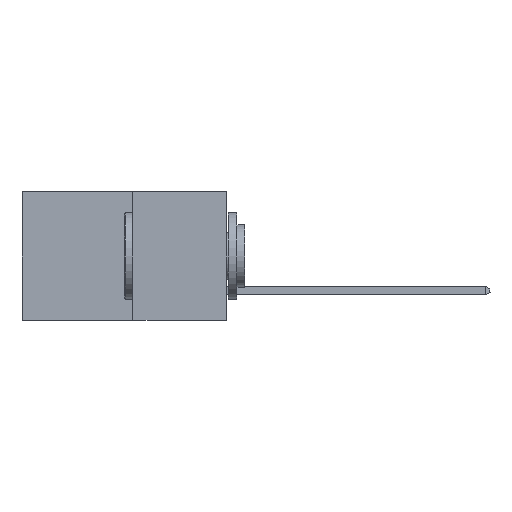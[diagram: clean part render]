
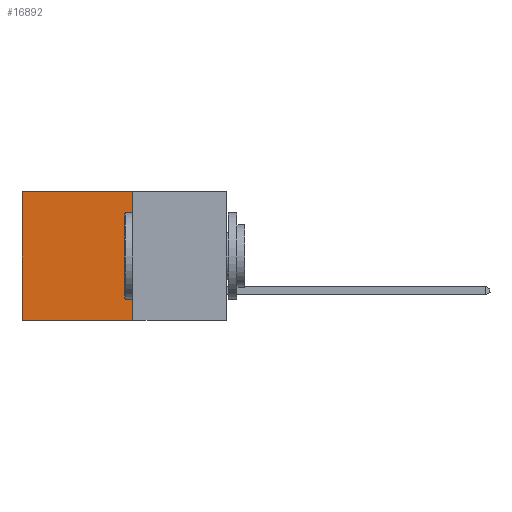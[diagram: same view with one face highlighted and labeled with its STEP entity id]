
A CAD part, left-side view. The second image highlights one B-rep face of the part: STEP entity #16892.
In plain terms, the highlighted planar face has unit normal (-1, 0, 0).
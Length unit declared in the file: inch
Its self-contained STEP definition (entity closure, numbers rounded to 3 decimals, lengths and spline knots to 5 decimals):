
#365 = VECTOR ( 'NONE', #19151, 39.37008 ) ;
#368 = CARTESIAN_POINT ( 'NONE',  ( 0.277, 0.59, 0. ) ) ;
#751 = FACE_OUTER_BOUND ( 'NONE', #15248, .T. ) ;
#902 = LINE ( 'NONE', #19407, #365 ) ;
#994 = CARTESIAN_POINT ( 'NONE',  ( 0.277, 0.27, -0.37 ) ) ;
#2076 = ORIENTED_EDGE ( 'NONE', *, *, #5922, .T. ) ;
#2740 = VECTOR ( 'NONE', #10110, 39.37008 ) ;
#2936 = CARTESIAN_POINT ( 'NONE',  ( 0.277, 0.59, -0.37 ) ) ;
#3285 = LINE ( 'NONE', #11860, #2740 ) ;
#3890 = LINE ( 'NONE', #19130, #8025 ) ;
#3902 = VERTEX_POINT ( 'NONE', #368 ) ;
#4713 = DIRECTION ( 'NONE',  ( 0., 0., -1. ) ) ;
#5631 = PLANE ( 'NONE',  #19453 ) ;
#5729 = VECTOR ( 'NONE', #4713, 39.37008 ) ;
#5922 = EDGE_CURVE ( 'NONE', #9801, #3902, #902, .T. ) ;
#7409 = DIRECTION ( 'NONE',  ( 1., 0., 0. ) ) ;
#7413 = VERTEX_POINT ( 'NONE', #19163 ) ;
#8025 = VECTOR ( 'NONE', #12296, 39.37008 ) ;
#8832 = VERTEX_POINT ( 'NONE', #994 ) ;
#9571 = EDGE_CURVE ( 'NONE', #3902, #7413, #10359, .T. ) ;
#9782 = ORIENTED_EDGE ( 'NONE', *, *, #15269, .F. ) ;
#9801 = VERTEX_POINT ( 'NONE', #20812 ) ;
#10110 = DIRECTION ( 'NONE',  ( 0., 1., 0. ) ) ;
#10359 = LINE ( 'NONE', #2936, #5729 ) ;
#10508 = ORIENTED_EDGE ( 'NONE', *, *, #9571, .T. ) ;
#11860 = CARTESIAN_POINT ( 'NONE',  ( 0.277, 0.27, -0.37 ) ) ;
#12296 = DIRECTION ( 'NONE',  ( 0., 0., -1. ) ) ;
#14237 = EDGE_CURVE ( 'NONE', #9801, #8832, #3890, .T. ) ;
#15248 = EDGE_LOOP ( 'NONE', ( #10508, #9782, #19873, #2076 ) ) ;
#15269 = EDGE_CURVE ( 'NONE', #8832, #7413, #3285, .T. ) ;
#16892 = ADVANCED_FACE ( 'NONE', ( #751 ), #5631, .F. ) ;
#17751 = CARTESIAN_POINT ( 'NONE',  ( 0.277, 0.27, -0.37 ) ) ;
#19130 = CARTESIAN_POINT ( 'NONE',  ( 0.277, 0.27, -0.37 ) ) ;
#19151 = DIRECTION ( 'NONE',  ( 0., 1., 0. ) ) ;
#19163 = CARTESIAN_POINT ( 'NONE',  ( 0.277, 0.59, -0.37 ) ) ;
#19407 = CARTESIAN_POINT ( 'NONE',  ( 0.277, 0.27, 0. ) ) ;
#19445 = DIRECTION ( 'NONE',  ( 0., 0., -1. ) ) ;
#19453 = AXIS2_PLACEMENT_3D ( 'NONE', #17751, #7409, #19445 ) ;
#19873 = ORIENTED_EDGE ( 'NONE', *, *, #14237, .F. ) ;
#20812 = CARTESIAN_POINT ( 'NONE',  ( 0.277, 0.27, 0. ) ) ;
